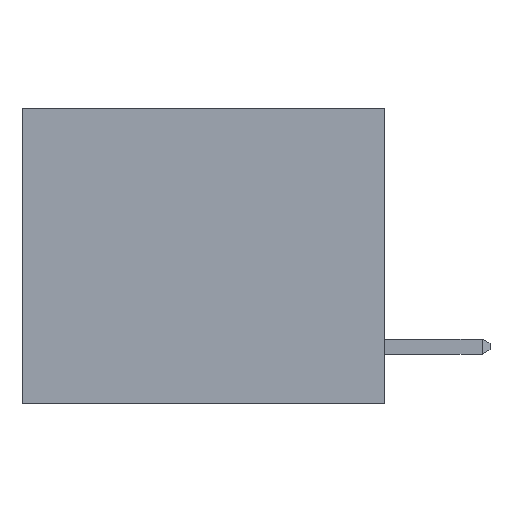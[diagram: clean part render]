
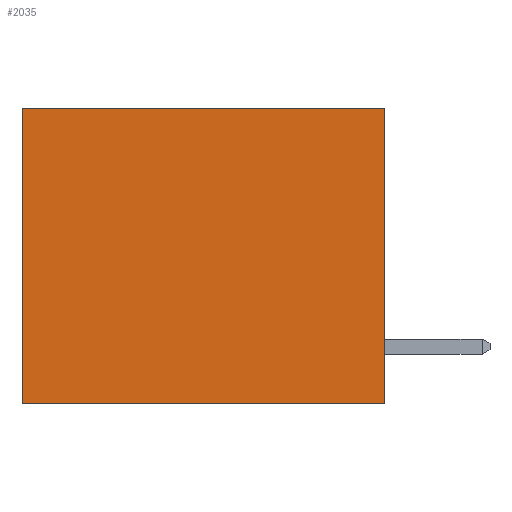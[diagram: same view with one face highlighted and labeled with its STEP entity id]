
A CAD part, left-side view. The second image highlights one B-rep face of the part: STEP entity #2035.
In plain terms, the highlighted planar face has unit normal (-1, 0, 0).
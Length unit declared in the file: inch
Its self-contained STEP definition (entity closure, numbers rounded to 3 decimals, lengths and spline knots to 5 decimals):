
#431 = CARTESIAN_POINT ( 'NONE',  ( 0.3165, 0.6, -0.49 ) ) ;
#466 = VERTEX_POINT ( 'NONE', #4105 ) ;
#473 = DIRECTION ( 'NONE',  ( 0., 0., -1. ) ) ;
#493 = EDGE_CURVE ( 'NONE', #8013, #466, #2803, .T. ) ;
#528 = PLANE ( 'NONE',  #1987 ) ;
#999 = VECTOR ( 'NONE', #4532, 39.37008 ) ;
#1055 = CARTESIAN_POINT ( 'NONE',  ( 0.3165, 0., 0. ) ) ;
#1226 = ORIENTED_EDGE ( 'NONE', *, *, #493, .T. ) ;
#1262 = CARTESIAN_POINT ( 'NONE',  ( 0.3165, 0., 0. ) ) ;
#1312 = CARTESIAN_POINT ( 'NONE',  ( 0.3165, 0., -0.49 ) ) ;
#1396 = LINE ( 'NONE', #3990, #999 ) ;
#1661 = ORIENTED_EDGE ( 'NONE', *, *, #6159, .T. ) ;
#1788 = DIRECTION ( 'NONE',  ( 0., 0., -1. ) ) ;
#1821 = VECTOR ( 'NONE', #5658, 39.37008 ) ;
#1839 = VECTOR ( 'NONE', #473, 39.37008 ) ;
#1984 = CARTESIAN_POINT ( 'NONE',  ( 0.3165, 0.6, -0.49 ) ) ;
#1987 = AXIS2_PLACEMENT_3D ( 'NONE', #5483, #5506, #1788 ) ;
#2035 = ADVANCED_FACE ( 'NONE', ( #2567 ), #528, .F. ) ;
#2312 = DIRECTION ( 'NONE',  ( 0., 1., 0. ) ) ;
#2507 = LINE ( 'NONE', #431, #1839 ) ;
#2567 = FACE_OUTER_BOUND ( 'NONE', #3973, .T. ) ;
#2803 = LINE ( 'NONE', #1055, #7335 ) ;
#2857 = EDGE_CURVE ( 'NONE', #8013, #5528, #1396, .T. ) ;
#3095 = ORIENTED_EDGE ( 'NONE', *, *, #7041, .F. ) ;
#3462 = LINE ( 'NONE', #1312, #1821 ) ;
#3973 = EDGE_LOOP ( 'NONE', ( #1661, #3095, #6769, #1226 ) ) ;
#3990 = CARTESIAN_POINT ( 'NONE',  ( 0.3165, 0., -0.49 ) ) ;
#4105 = CARTESIAN_POINT ( 'NONE',  ( 0.3165, 0.6, 0. ) ) ;
#4532 = DIRECTION ( 'NONE',  ( 0., 0., -1. ) ) ;
#5483 = CARTESIAN_POINT ( 'NONE',  ( 0.3165, 0., -0.49 ) ) ;
#5506 = DIRECTION ( 'NONE',  ( 1., 0., 0. ) ) ;
#5528 = VERTEX_POINT ( 'NONE', #7297 ) ;
#5658 = DIRECTION ( 'NONE',  ( 0., 1., 0. ) ) ;
#6159 = EDGE_CURVE ( 'NONE', #466, #7077, #2507, .T. ) ;
#6769 = ORIENTED_EDGE ( 'NONE', *, *, #2857, .F. ) ;
#7041 = EDGE_CURVE ( 'NONE', #5528, #7077, #3462, .T. ) ;
#7077 = VERTEX_POINT ( 'NONE', #1984 ) ;
#7297 = CARTESIAN_POINT ( 'NONE',  ( 0.3165, 0., -0.49 ) ) ;
#7335 = VECTOR ( 'NONE', #2312, 39.37008 ) ;
#8013 = VERTEX_POINT ( 'NONE', #1262 ) ;
